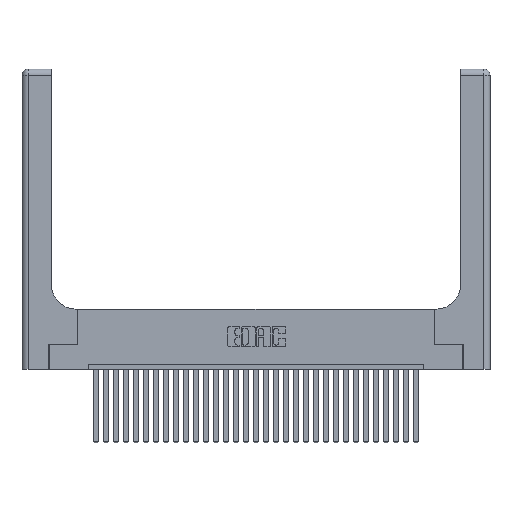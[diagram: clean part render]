
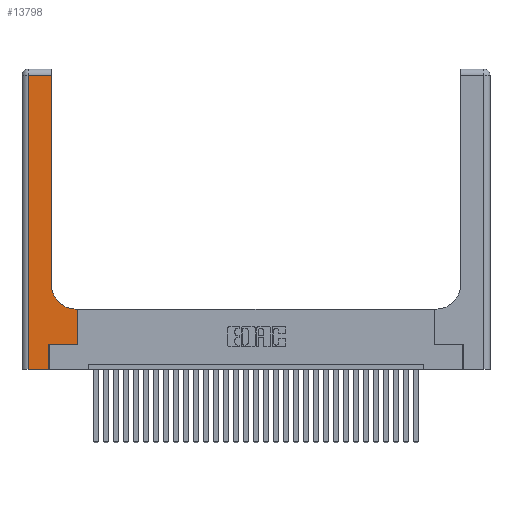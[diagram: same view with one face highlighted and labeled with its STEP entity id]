
A CAD part, top view. The second image highlights one B-rep face of the part: STEP entity #13798.
In plain terms, the highlighted planar face has unit normal (0, 0, 1).
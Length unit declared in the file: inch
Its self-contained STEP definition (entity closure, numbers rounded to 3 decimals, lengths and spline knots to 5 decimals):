
#44 = FACE_OUTER_BOUND ( 'NONE', #7922, .T. ) ;
#997 = ORIENTED_EDGE ( 'NONE', *, *, #27581, .T. ) ;
#1219 = CIRCLE ( 'NONE', #3072, 0.25 ) ;
#1424 = LINE ( 'NONE', #3558, #20164 ) ;
#1471 = LINE ( 'NONE', #10682, #3312 ) ;
#1714 = ORIENTED_EDGE ( 'NONE', *, *, #12958, .T. ) ;
#1945 = VECTOR ( 'NONE', #30290, 39.37008 ) ;
#2190 = CARTESIAN_POINT ( 'NONE',  ( 0.2915, 2.94, 0.37 ) ) ;
#2349 = VECTOR ( 'NONE', #9622, 39.37008 ) ;
#2708 = CARTESIAN_POINT ( 'NONE',  ( 0.269, 0.25, 0.37 ) ) ;
#3072 = AXIS2_PLACEMENT_3D ( 'NONE', #30911, #23912, #16422 ) ;
#3312 = VECTOR ( 'NONE', #22608, 39.37008 ) ;
#3417 = DIRECTION ( 'NONE',  ( 0., 0., -1. ) ) ;
#3558 = CARTESIAN_POINT ( 'NONE',  ( 0., 0., 0.37 ) ) ;
#3670 = VERTEX_POINT ( 'NONE', #18171 ) ;
#3858 = ORIENTED_EDGE ( 'NONE', *, *, #11921, .T. ) ;
#3901 = LINE ( 'NONE', #14220, #21535 ) ;
#4517 = VECTOR ( 'NONE', #21612, 39.37008 ) ;
#4892 = CARTESIAN_POINT ( 'NONE',  ( 0., 2.94, 0.37 ) ) ;
#5764 = DIRECTION ( 'NONE',  ( 1., 0., 0. ) ) ;
#6056 = LINE ( 'NONE', #2708, #20699 ) ;
#7370 = ORIENTED_EDGE ( 'NONE', *, *, #20647, .T. ) ;
#7601 = LINE ( 'NONE', #4892, #2349 ) ;
#7922 = EDGE_LOOP ( 'NONE', ( #15809, #7370, #3858, #21426, #29412, #15052, #997, #1714, #17365 ) ) ;
#8027 = VERTEX_POINT ( 'NONE', #17154 ) ;
#8772 = CARTESIAN_POINT ( 'NONE',  ( 0.06, 3., 0.37 ) ) ;
#9066 = AXIS2_PLACEMENT_3D ( 'NONE', #17782, #3417, #29389 ) ;
#9333 = VERTEX_POINT ( 'NONE', #23618 ) ;
#9622 = DIRECTION ( 'NONE',  ( -1., 0., 0. ) ) ;
#10035 = EDGE_CURVE ( 'NONE', #28849, #26665, #1471, .T. ) ;
#10682 = CARTESIAN_POINT ( 'NONE',  ( 0.269, 0., 0.37 ) ) ;
#10936 = CARTESIAN_POINT ( 'NONE',  ( 0.06, 0., 0.37 ) ) ;
#11192 = DIRECTION ( 'NONE',  ( 0., -1., 0. ) ) ;
#11921 = EDGE_CURVE ( 'NONE', #9333, #25733, #13717, .T. ) ;
#12958 = EDGE_CURVE ( 'NONE', #27940, #26156, #3901, .T. ) ;
#13324 = VECTOR ( 'NONE', #11192, 39.37008 ) ;
#13717 = LINE ( 'NONE', #8772, #13324 ) ;
#13798 = ADVANCED_FACE ( 'NONE', ( #44 ), #24541, .F. ) ;
#14011 = EDGE_CURVE ( 'NONE', #8027, #25200, #30733, .T. ) ;
#14220 = CARTESIAN_POINT ( 'NONE',  ( 0.2915, 0.6, 0.37 ) ) ;
#14346 = DIRECTION ( 'NONE',  ( 1., 0., 0. ) ) ;
#15052 = ORIENTED_EDGE ( 'NONE', *, *, #21567, .T. ) ;
#15153 = CARTESIAN_POINT ( 'NONE',  ( 0.269, 0., 0.37 ) ) ;
#15809 = ORIENTED_EDGE ( 'NONE', *, *, #14011, .T. ) ;
#16242 = LINE ( 'NONE', #25465, #1945 ) ;
#16422 = DIRECTION ( 'NONE',  ( 1., 0., 0. ) ) ;
#16565 = DIRECTION ( 'NONE',  ( -1., 0., 0. ) ) ;
#16617 = CARTESIAN_POINT ( 'NONE',  ( 0.2915, 3., 0.37 ) ) ;
#17154 = CARTESIAN_POINT ( 'NONE',  ( 0.2915, 0.85, 0.37 ) ) ;
#17365 = ORIENTED_EDGE ( 'NONE', *, *, #27152, .T. ) ;
#17782 = CARTESIAN_POINT ( 'NONE',  ( 0., 3., 0.37 ) ) ;
#17819 = CARTESIAN_POINT ( 'NONE',  ( 0.5585, 0.6, 0.37 ) ) ;
#18171 = CARTESIAN_POINT ( 'NONE',  ( 0.5585, 0.25, 0.37 ) ) ;
#20164 = VECTOR ( 'NONE', #5764, 39.37008 ) ;
#20647 = EDGE_CURVE ( 'NONE', #25200, #9333, #7601, .T. ) ;
#20699 = VECTOR ( 'NONE', #14346, 39.37008 ) ;
#21426 = ORIENTED_EDGE ( 'NONE', *, *, #23005, .T. ) ;
#21535 = VECTOR ( 'NONE', #16565, 39.37008 ) ;
#21567 = EDGE_CURVE ( 'NONE', #26665, #3670, #6056, .T. ) ;
#21612 = DIRECTION ( 'NONE',  ( 0., 1., 0. ) ) ;
#22072 = CARTESIAN_POINT ( 'NONE',  ( 0.269, 0.25, 0.37 ) ) ;
#22608 = DIRECTION ( 'NONE',  ( 0., 1., 0. ) ) ;
#23005 = EDGE_CURVE ( 'NONE', #25733, #28849, #1424, .T. ) ;
#23618 = CARTESIAN_POINT ( 'NONE',  ( 0.06, 2.94, 0.37 ) ) ;
#23912 = DIRECTION ( 'NONE',  ( 0., 0., -1. ) ) ;
#24541 = PLANE ( 'NONE',  #9066 ) ;
#25200 = VERTEX_POINT ( 'NONE', #2190 ) ;
#25465 = CARTESIAN_POINT ( 'NONE',  ( 0.5585, 0.25, 0.37 ) ) ;
#25733 = VERTEX_POINT ( 'NONE', #10936 ) ;
#26156 = VERTEX_POINT ( 'NONE', #27510 ) ;
#26665 = VERTEX_POINT ( 'NONE', #22072 ) ;
#27152 = EDGE_CURVE ( 'NONE', #26156, #8027, #1219, .T. ) ;
#27510 = CARTESIAN_POINT ( 'NONE',  ( 0.5415, 0.6, 0.37 ) ) ;
#27581 = EDGE_CURVE ( 'NONE', #3670, #27940, #16242, .T. ) ;
#27940 = VERTEX_POINT ( 'NONE', #17819 ) ;
#28849 = VERTEX_POINT ( 'NONE', #15153 ) ;
#29389 = DIRECTION ( 'NONE',  ( -1., 0., 0. ) ) ;
#29412 = ORIENTED_EDGE ( 'NONE', *, *, #10035, .T. ) ;
#30290 = DIRECTION ( 'NONE',  ( 0., 1., 0. ) ) ;
#30733 = LINE ( 'NONE', #16617, #4517 ) ;
#30911 = CARTESIAN_POINT ( 'NONE',  ( 0.5415, 0.85, 0.37 ) ) ;
